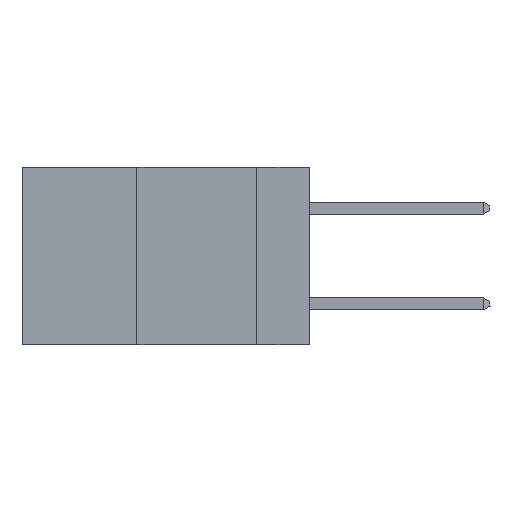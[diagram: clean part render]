
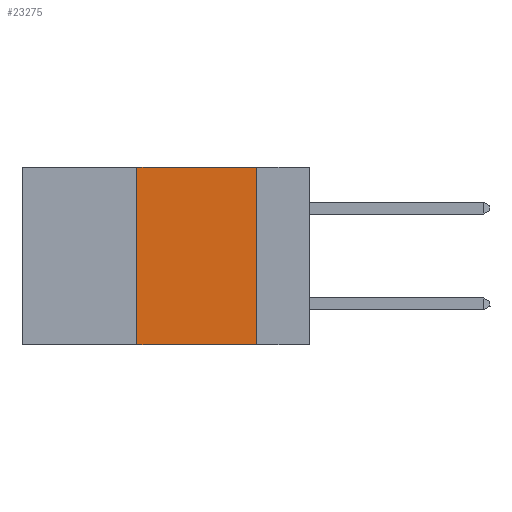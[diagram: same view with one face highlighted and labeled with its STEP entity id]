
A CAD part, left-side view. The second image highlights one B-rep face of the part: STEP entity #23275.
In plain terms, the highlighted planar face has unit normal (-1, 0, 0).
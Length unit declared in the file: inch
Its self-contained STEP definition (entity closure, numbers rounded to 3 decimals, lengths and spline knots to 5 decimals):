
#64 = ORIENTED_EDGE ( 'NONE', *, *, #5266, .F. ) ;
#150 = VECTOR ( 'NONE', #24560, 39.37008 ) ;
#4358 = VERTEX_POINT ( 'NONE', #12081 ) ;
#4394 = DIRECTION ( 'NONE',  ( 0., 0., 1. ) ) ;
#4451 = DIRECTION ( 'NONE',  ( 1., 0., 0. ) ) ;
#4877 = ORIENTED_EDGE ( 'NONE', *, *, #11855, .T. ) ;
#5266 = EDGE_CURVE ( 'NONE', #4358, #6452, #20770, .T. ) ;
#5669 = CARTESIAN_POINT ( 'NONE',  ( 0., 0.6, -0.37 ) ) ;
#5724 = VECTOR ( 'NONE', #4394, 39.37008 ) ;
#5868 = EDGE_CURVE ( 'NONE', #6935, #4358, #14443, .T. ) ;
#6452 = VERTEX_POINT ( 'NONE', #27059 ) ;
#6678 = CARTESIAN_POINT ( 'NONE',  ( 0., 0.11, 0. ) ) ;
#6935 = VERTEX_POINT ( 'NONE', #25081 ) ;
#7547 = DIRECTION ( 'NONE',  ( 0., 0., -1. ) ) ;
#9573 = PLANE ( 'NONE',  #11817 ) ;
#9847 = ORIENTED_EDGE ( 'NONE', *, *, #10956, .F. ) ;
#10635 = EDGE_LOOP ( 'NONE', ( #64, #12261, #9847, #4877 ) ) ;
#10956 = EDGE_CURVE ( 'NONE', #30447, #6935, #14227, .T. ) ;
#11817 = AXIS2_PLACEMENT_3D ( 'NONE', #25793, #4451, #11871 ) ;
#11855 = EDGE_CURVE ( 'NONE', #30447, #6452, #21177, .T. ) ;
#11871 = DIRECTION ( 'NONE',  ( 0., 0., -1. ) ) ;
#12057 = DIRECTION ( 'NONE',  ( 0., -1., 0. ) ) ;
#12081 = CARTESIAN_POINT ( 'NONE',  ( 0., 0.11, 0. ) ) ;
#12261 = ORIENTED_EDGE ( 'NONE', *, *, #5868, .F. ) ;
#14227 = LINE ( 'NONE', #23379, #5724 ) ;
#14443 = LINE ( 'NONE', #21188, #28094 ) ;
#18341 = FACE_OUTER_BOUND ( 'NONE', #10635, .T. ) ;
#19241 = VECTOR ( 'NONE', #7547, 39.37008 ) ;
#20770 = LINE ( 'NONE', #6678, #19241 ) ;
#21177 = LINE ( 'NONE', #5669, #150 ) ;
#21188 = CARTESIAN_POINT ( 'NONE',  ( 0., 0.6, 0. ) ) ;
#23275 = ADVANCED_FACE ( 'NONE', ( #18341 ), #9573, .F. ) ;
#23379 = CARTESIAN_POINT ( 'NONE',  ( 0., 0.36, 0. ) ) ;
#24560 = DIRECTION ( 'NONE',  ( 0., -1., 0. ) ) ;
#25081 = CARTESIAN_POINT ( 'NONE',  ( 0., 0.36, 0. ) ) ;
#25793 = CARTESIAN_POINT ( 'NONE',  ( 0., 0.6, 0. ) ) ;
#27001 = CARTESIAN_POINT ( 'NONE',  ( 0., 0.36, -0.37 ) ) ;
#27059 = CARTESIAN_POINT ( 'NONE',  ( 0., 0.11, -0.37 ) ) ;
#28094 = VECTOR ( 'NONE', #12057, 39.37008 ) ;
#30447 = VERTEX_POINT ( 'NONE', #27001 ) ;
